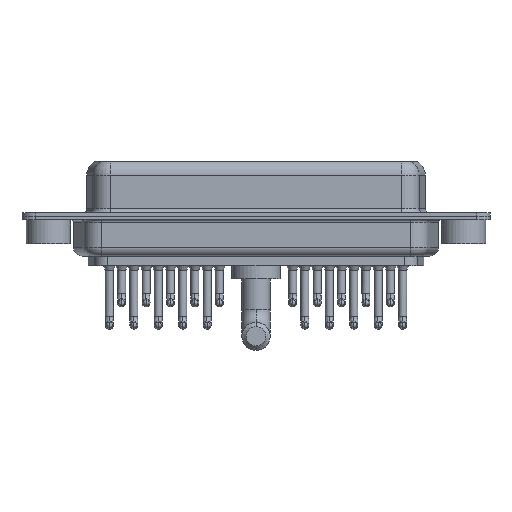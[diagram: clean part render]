
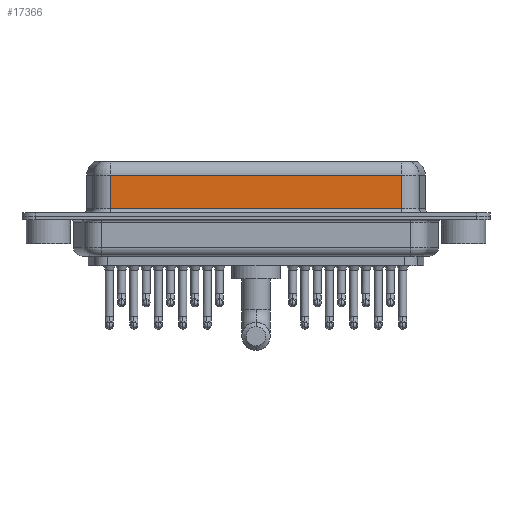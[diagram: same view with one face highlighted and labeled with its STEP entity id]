
A CAD part, front view. The second image highlights one B-rep face of the part: STEP entity #17366.
In plain terms, the highlighted planar face has unit normal (0, -1, 0).
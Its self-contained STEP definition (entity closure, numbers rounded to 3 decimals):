
#752 = EDGE_LOOP ( 'NONE', ( #11286, #4743, #13535, #21997 ) ) ;
#2423 = LINE ( 'NONE', #16423, #8194 ) ;
#3366 = PLANE ( 'NONE',  #7161 ) ;
#3819 = EDGE_CURVE ( 'NONE', #21416, #21390, #22227, .T. ) ;
#3907 = VERTEX_POINT ( 'NONE', #5375 ) ;
#4743 = ORIENTED_EDGE ( 'NONE', *, *, #11630, .T. ) ;
#4801 = DIRECTION ( 'NONE',  ( -1., 0., 0. ) ) ;
#4928 = CARTESIAN_POINT ( 'NONE',  ( 40.037, -3.95, 4.65 ) ) ;
#5375 = CARTESIAN_POINT ( 'NONE',  ( 7.013, -3.95, 0.9 ) ) ;
#6818 = FACE_OUTER_BOUND ( 'NONE', #752, .T. ) ;
#7161 = AXIS2_PLACEMENT_3D ( 'NONE', #10381, #8659, #10952 ) ;
#8075 = VECTOR ( 'NONE', #4801, 1000. ) ;
#8194 = VECTOR ( 'NONE', #16755, 1000. ) ;
#8498 = DIRECTION ( 'NONE',  ( 0., 0., -1. ) ) ;
#8659 = DIRECTION ( 'NONE',  ( 0., 1., 0. ) ) ;
#10381 = CARTESIAN_POINT ( 'NONE',  ( 40.037, -3.95, 6.4 ) ) ;
#10642 = VERTEX_POINT ( 'NONE', #13647 ) ;
#10952 = DIRECTION ( 'NONE',  ( 0., 0., 1. ) ) ;
#11286 = ORIENTED_EDGE ( 'NONE', *, *, #3819, .F. ) ;
#11579 = CARTESIAN_POINT ( 'NONE',  ( 40.037, -3.95, 6.4 ) ) ;
#11630 = EDGE_CURVE ( 'NONE', #21416, #10642, #19272, .T. ) ;
#13535 = ORIENTED_EDGE ( 'NONE', *, *, #15686, .T. ) ;
#13647 = CARTESIAN_POINT ( 'NONE',  ( 7.013, -3.95, 4.65 ) ) ;
#15156 = CARTESIAN_POINT ( 'NONE',  ( 7.013, -3.95, 6.4 ) ) ;
#15686 = EDGE_CURVE ( 'NONE', #10642, #3907, #20446, .T. ) ;
#15951 = VECTOR ( 'NONE', #22332, 1000. ) ;
#16423 = CARTESIAN_POINT ( 'NONE',  ( 40.037, -3.95, 0.9 ) ) ;
#16755 = DIRECTION ( 'NONE',  ( 1., 0., 0. ) ) ;
#17226 = CARTESIAN_POINT ( 'NONE',  ( 40.037, -3.95, 4.65 ) ) ;
#17340 = VECTOR ( 'NONE', #8498, 1000. ) ;
#17366 = ADVANCED_FACE ( 'NONE', ( #6818 ), #3366, .F. ) ;
#19272 = LINE ( 'NONE', #4928, #8075 ) ;
#20446 = LINE ( 'NONE', #15156, #17340 ) ;
#20556 = CARTESIAN_POINT ( 'NONE',  ( 40.037, -3.95, 0.9 ) ) ;
#21390 = VERTEX_POINT ( 'NONE', #20556 ) ;
#21416 = VERTEX_POINT ( 'NONE', #17226 ) ;
#21706 = EDGE_CURVE ( 'NONE', #3907, #21390, #2423, .T. ) ;
#21997 = ORIENTED_EDGE ( 'NONE', *, *, #21706, .T. ) ;
#22227 = LINE ( 'NONE', #11579, #15951 ) ;
#22332 = DIRECTION ( 'NONE',  ( 0., 0., -1. ) ) ;
